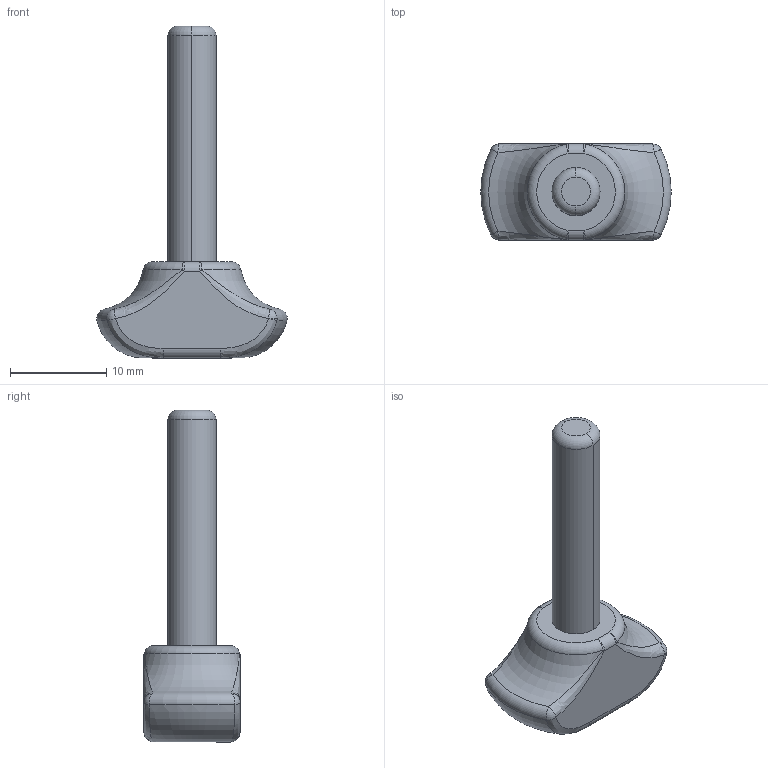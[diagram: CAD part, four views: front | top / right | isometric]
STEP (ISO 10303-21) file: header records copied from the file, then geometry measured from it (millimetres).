
FILE_DESCRIPTION (( 'STEP AP214' ), '1' );
FILE_NAME ('Plunger_Pin.STEP', '2013-09-01T16:40:05', ( 'Asher' ), ( '' ), 'SwSTEP 2.0', 'SolidWorks 2013', '' );
FILE_SCHEMA (( 'AUTOMOTIVE_DESIGN' ));
Length unit declared in the file: millimetre
Products named in the file (1): Plunger_Pin
Bounding box: 19.79 x 10 x 34.5 mm (x, y, z)
Volume: 1826 mm3; surface area: 1064.5 mm2
Topology: 1 solids, 1 shells, 39 faces, 80 edges, 40 vertices
Faces by surface type: torus 10, sphere 10, bspline 8, cylinder 6, plane 5
Entity records: 1494 total; most frequent: CARTESIAN_POINT 696, DIRECTION 174, ORIENTED_EDGE 152, AXIS2_PLACEMENT_3D 82, EDGE_CURVE 76, CIRCLE 50, VERTEX_POINT 40, EDGE_LOOP 40
